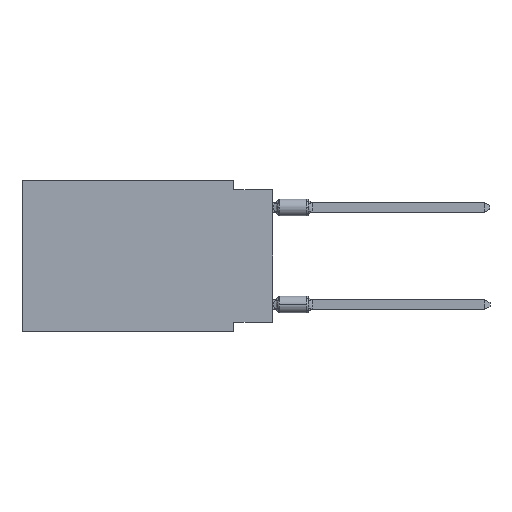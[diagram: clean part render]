
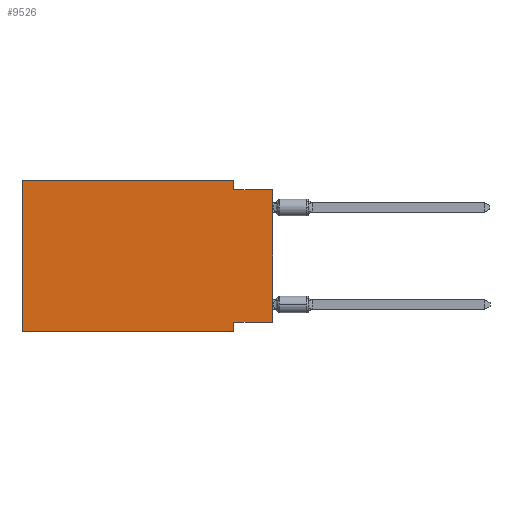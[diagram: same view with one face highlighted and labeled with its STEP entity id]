
A CAD part, left-side view. The second image highlights one B-rep face of the part: STEP entity #9526.
In plain terms, the highlighted planar face has unit normal (-1, 0, 0).
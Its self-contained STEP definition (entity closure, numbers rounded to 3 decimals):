
#119 = ORIENTED_EDGE ( 'NONE', *, *, #3602, .T. ) ;
#232 = EDGE_CURVE ( 'NONE', #7555, #5067, #1547, .T. ) ;
#387 = LINE ( 'NONE', #4362, #5790 ) ;
#840 = CARTESIAN_POINT ( 'NONE',  ( 0., 16.383, 0. ) ) ;
#855 = CARTESIAN_POINT ( 'NONE',  ( 0., 16.383, 0. ) ) ;
#889 = DIRECTION ( 'NONE',  ( 1., 0., 0. ) ) ;
#1006 = DIRECTION ( 'NONE',  ( 0., 0., -1. ) ) ;
#1543 = VERTEX_POINT ( 'NONE', #1676 ) ;
#1547 = LINE ( 'NONE', #11648, #4000 ) ;
#1676 = CARTESIAN_POINT ( 'NONE',  ( 0., 16.383, -9.906 ) ) ;
#1831 = CARTESIAN_POINT ( 'NONE',  ( 0., 0., -9.271 ) ) ;
#2276 = VERTEX_POINT ( 'NONE', #10700 ) ;
#2724 = LINE ( 'NONE', #2921, #9349 ) ;
#2835 = CARTESIAN_POINT ( 'NONE',  ( 0., 2.54, 0. ) ) ;
#2836 = VERTEX_POINT ( 'NONE', #4666 ) ;
#2921 = CARTESIAN_POINT ( 'NONE',  ( 0., 16.383, -9.906 ) ) ;
#3264 = VECTOR ( 'NONE', #1006, 1000. ) ;
#3284 = VERTEX_POINT ( 'NONE', #7758 ) ;
#3602 = EDGE_CURVE ( 'NONE', #7555, #8430, #7682, .T. ) ;
#3888 = CARTESIAN_POINT ( 'NONE',  ( 0., 0., -0.635 ) ) ;
#3906 = DIRECTION ( 'NONE',  ( 0., -1., 0. ) ) ;
#4000 = VECTOR ( 'NONE', #5406, 1000. ) ;
#4362 = CARTESIAN_POINT ( 'NONE',  ( 0., 0., -0.635 ) ) ;
#4434 = CARTESIAN_POINT ( 'NONE',  ( 0., 2.54, -9.906 ) ) ;
#4482 = VECTOR ( 'NONE', #8699, 1000. ) ;
#4666 = CARTESIAN_POINT ( 'NONE',  ( 0., 2.54, -0.635 ) ) ;
#4870 = CARTESIAN_POINT ( 'NONE',  ( 0., 16.383, 0. ) ) ;
#4984 = EDGE_LOOP ( 'NONE', ( #119, #8073, #5430, #12283, #5065, #11551, #5508, #5627 ) ) ;
#4993 = DIRECTION ( 'NONE',  ( 0., 0., -1. ) ) ;
#5065 = ORIENTED_EDGE ( 'NONE', *, *, #6023, .F. ) ;
#5067 = VERTEX_POINT ( 'NONE', #10361 ) ;
#5143 = VECTOR ( 'NONE', #3906, 1000. ) ;
#5329 = AXIS2_PLACEMENT_3D ( 'NONE', #4870, #889, #4993 ) ;
#5406 = DIRECTION ( 'NONE',  ( 0., 1., 0. ) ) ;
#5430 = ORIENTED_EDGE ( 'NONE', *, *, #9965, .F. ) ;
#5508 = ORIENTED_EDGE ( 'NONE', *, *, #9400, .F. ) ;
#5555 = EDGE_CURVE ( 'NONE', #2836, #8430, #387, .T. ) ;
#5627 = ORIENTED_EDGE ( 'NONE', *, *, #232, .F. ) ;
#5790 = VECTOR ( 'NONE', #9300, 1000. ) ;
#5944 = DIRECTION ( 'NONE',  ( 0., -1., 0. ) ) ;
#6023 = EDGE_CURVE ( 'NONE', #1543, #2276, #9787, .T. ) ;
#6358 = EDGE_CURVE ( 'NONE', #1543, #7861, #2724, .T. ) ;
#6656 = CARTESIAN_POINT ( 'NONE',  ( 0., 2.54, -9.906 ) ) ;
#7555 = VERTEX_POINT ( 'NONE', #1831 ) ;
#7682 = LINE ( 'NONE', #12908, #11952 ) ;
#7758 = CARTESIAN_POINT ( 'NONE',  ( 0., 2.54, 0. ) ) ;
#7861 = VERTEX_POINT ( 'NONE', #4434 ) ;
#8073 = ORIENTED_EDGE ( 'NONE', *, *, #5555, .F. ) ;
#8118 = EDGE_CURVE ( 'NONE', #2276, #3284, #9766, .T. ) ;
#8430 = VERTEX_POINT ( 'NONE', #3888 ) ;
#8699 = DIRECTION ( 'NONE',  ( 0., 0., -1. ) ) ;
#9300 = DIRECTION ( 'NONE',  ( 0., -1., 0. ) ) ;
#9349 = VECTOR ( 'NONE', #5944, 1000. ) ;
#9400 = EDGE_CURVE ( 'NONE', #5067, #7861, #12507, .T. ) ;
#9526 = ADVANCED_FACE ( 'NONE', ( #11066 ), #11784, .F. ) ;
#9766 = LINE ( 'NONE', #840, #5143 ) ;
#9787 = LINE ( 'NONE', #855, #11229 ) ;
#9965 = EDGE_CURVE ( 'NONE', #3284, #2836, #12026, .T. ) ;
#10361 = CARTESIAN_POINT ( 'NONE',  ( 0., 2.54, -9.271 ) ) ;
#10700 = CARTESIAN_POINT ( 'NONE',  ( 0., 16.383, 0. ) ) ;
#11034 = DIRECTION ( 'NONE',  ( 0., 0., 1. ) ) ;
#11066 = FACE_OUTER_BOUND ( 'NONE', #4984, .T. ) ;
#11229 = VECTOR ( 'NONE', #11034, 1000. ) ;
#11551 = ORIENTED_EDGE ( 'NONE', *, *, #6358, .T. ) ;
#11648 = CARTESIAN_POINT ( 'NONE',  ( 0., 0., -9.271 ) ) ;
#11685 = DIRECTION ( 'NONE',  ( 0., 0., 1. ) ) ;
#11784 = PLANE ( 'NONE',  #5329 ) ;
#11952 = VECTOR ( 'NONE', #11685, 1000. ) ;
#12026 = LINE ( 'NONE', #2835, #3264 ) ;
#12283 = ORIENTED_EDGE ( 'NONE', *, *, #8118, .F. ) ;
#12507 = LINE ( 'NONE', #6656, #4482 ) ;
#12908 = CARTESIAN_POINT ( 'NONE',  ( 0., 0., 0. ) ) ;
